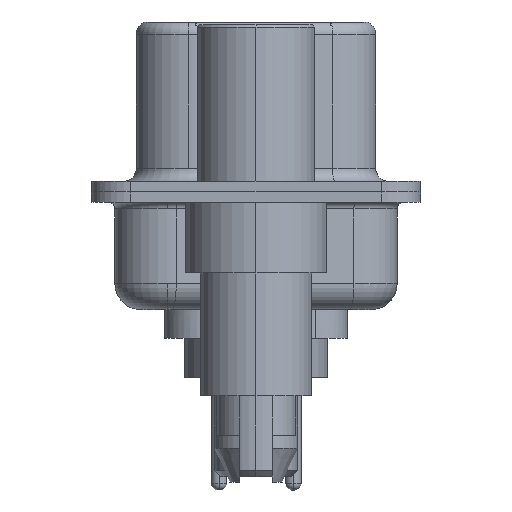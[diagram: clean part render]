
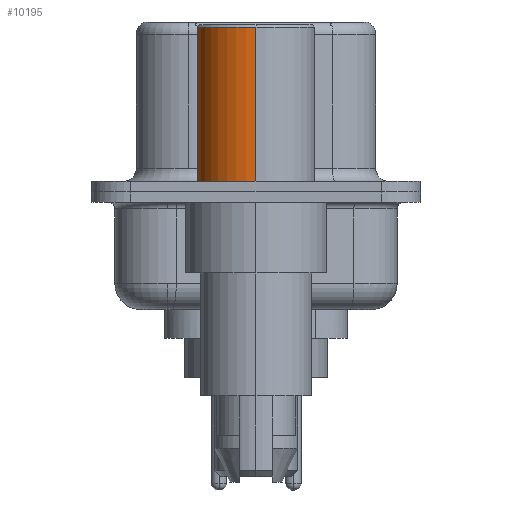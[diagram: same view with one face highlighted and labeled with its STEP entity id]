
A CAD part, left-side view. The second image highlights one B-rep face of the part: STEP entity #10195.
In plain terms, the highlighted cylindrical face has radius 2.25 mm (diameter 4.5 mm), a partial arc.
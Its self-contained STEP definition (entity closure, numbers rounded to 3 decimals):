
#582 = CARTESIAN_POINT ( 'NONE',  ( -2.25, 0., 0.4 ) ) ;
#1205 = CIRCLE ( 'NONE', #17715, 2.25 ) ;
#1214 = EDGE_CURVE ( 'NONE', #1336, #3099, #8900, .T. ) ;
#1336 = VERTEX_POINT ( 'NONE', #582 ) ;
#1999 = CIRCLE ( 'NONE', #17995, 2.25 ) ;
#2319 = VERTEX_POINT ( 'NONE', #21266 ) ;
#3099 = VERTEX_POINT ( 'NONE', #7933 ) ;
#3412 = CARTESIAN_POINT ( 'NONE',  ( -2.25, 0., 0.581 ) ) ;
#3473 = DIRECTION ( 'NONE',  ( 0., 0., 1. ) ) ;
#3946 = VECTOR ( 'NONE', #3473, 1000. ) ;
#4919 = EDGE_CURVE ( 'NONE', #9302, #1336, #1205, .T. ) ;
#6128 = CYLINDRICAL_SURFACE ( 'NONE', #9489, 2.25 ) ;
#6725 = FACE_OUTER_BOUND ( 'NONE', #7366, .T. ) ;
#6919 = ORIENTED_EDGE ( 'NONE', *, *, #12344, .F. ) ;
#7205 = DIRECTION ( 'NONE',  ( 0., 0., 1. ) ) ;
#7366 = EDGE_LOOP ( 'NONE', ( #13462, #11521, #6919, #21164 ) ) ;
#7694 = DIRECTION ( 'NONE',  ( 0., 0., 1. ) ) ;
#7933 = CARTESIAN_POINT ( 'NONE',  ( -2.25, 0., 6.3 ) ) ;
#8223 = DIRECTION ( 'NONE',  ( 1., 0., 0. ) ) ;
#8900 = LINE ( 'NONE', #3412, #3946 ) ;
#9302 = VERTEX_POINT ( 'NONE', #14399 ) ;
#9489 = AXIS2_PLACEMENT_3D ( 'NONE', #11298, #22255, #11447 ) ;
#10195 = ADVANCED_FACE ( 'NONE', ( #6725 ), #6128, .T. ) ;
#10633 = CARTESIAN_POINT ( 'NONE',  ( 0., 0., 6.3 ) ) ;
#11298 = CARTESIAN_POINT ( 'NONE',  ( 0., 0., 0.581 ) ) ;
#11447 = DIRECTION ( 'NONE',  ( 1., 0., 0. ) ) ;
#11521 = ORIENTED_EDGE ( 'NONE', *, *, #1214, .T. ) ;
#12344 = EDGE_CURVE ( 'NONE', #2319, #3099, #1999, .T. ) ;
#12461 = DIRECTION ( 'NONE',  ( 1., 0., 0. ) ) ;
#13462 = ORIENTED_EDGE ( 'NONE', *, *, #4919, .T. ) ;
#14188 = VECTOR ( 'NONE', #7205, 1000. ) ;
#14399 = CARTESIAN_POINT ( 'NONE',  ( 2.25, 0., 0.4 ) ) ;
#14751 = LINE ( 'NONE', #16290, #14188 ) ;
#16290 = CARTESIAN_POINT ( 'NONE',  ( 2.25, 0., 0.581 ) ) ;
#17715 = AXIS2_PLACEMENT_3D ( 'NONE', #18085, #7694, #8223 ) ;
#17995 = AXIS2_PLACEMENT_3D ( 'NONE', #10633, #23291, #12461 ) ;
#18085 = CARTESIAN_POINT ( 'NONE',  ( 0., 0., 0.4 ) ) ;
#21164 = ORIENTED_EDGE ( 'NONE', *, *, #21251, .F. ) ;
#21251 = EDGE_CURVE ( 'NONE', #9302, #2319, #14751, .T. ) ;
#21266 = CARTESIAN_POINT ( 'NONE',  ( 2.25, 0., 6.3 ) ) ;
#22255 = DIRECTION ( 'NONE',  ( 0., 0., 1. ) ) ;
#23291 = DIRECTION ( 'NONE',  ( 0., 0., 1. ) ) ;
